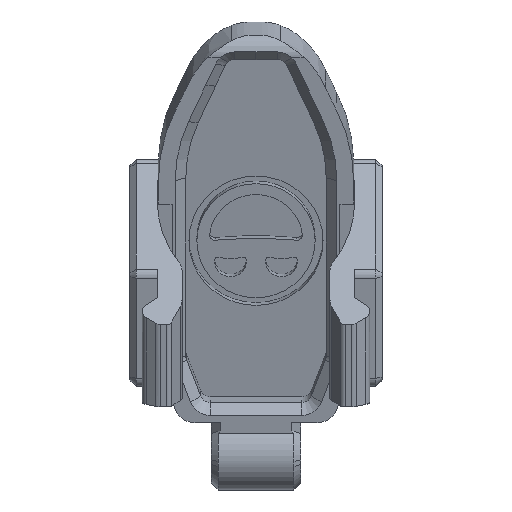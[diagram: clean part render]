
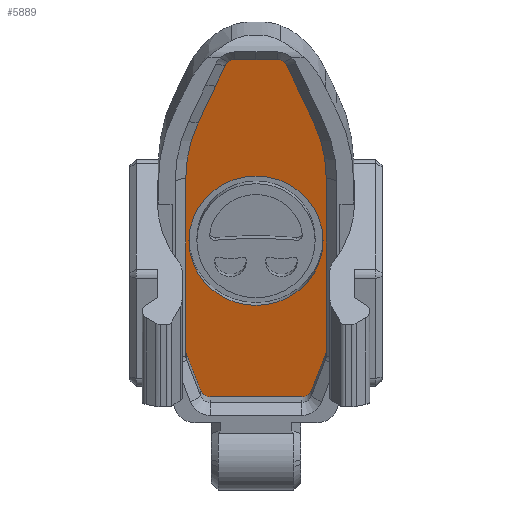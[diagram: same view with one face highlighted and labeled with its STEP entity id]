
A CAD part, top view. The second image highlights one B-rep face of the part: STEP entity #5889.
In plain terms, the highlighted planar face has unit normal (0, -0.266, 0.964).
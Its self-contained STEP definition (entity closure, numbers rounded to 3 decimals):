
#288=B_SPLINE_CURVE_WITH_KNOTS('',3,(#9458,#9459,#9460,#9461,#9462,#9463),
 .UNSPECIFIED.,.F.,.F.,(4,2,4),(0.,0.198,0.396),
 .UNSPECIFIED.);
#292=B_SPLINE_CURVE_WITH_KNOTS('',3,(#9488,#9489,#9490,#9491),
 .UNSPECIFIED.,.F.,.F.,(4,4),(-1.571,-1.141),
 .UNSPECIFIED.);
#359=B_SPLINE_CURVE_WITH_KNOTS('',3,(#11507,#11508,#11509,#11510,#11511,
#11512),.UNSPECIFIED.,.F.,.F.,(4,2,4),(0.,0.198,0.396),
 .UNSPECIFIED.);
#362=B_SPLINE_CURVE_WITH_KNOTS('',3,(#11533,#11534,#11535,#11536),
 .UNSPECIFIED.,.F.,.F.,(4,4),(-1.571,-1.141),
 .UNSPECIFIED.);
#551=LINE('',#9436,#1043);
#553=LINE('',#9494,#1045);
#557=LINE('',#9506,#1049);
#805=LINE('',#11489,#1297);
#809=LINE('',#11546,#1301);
#811=LINE('',#11555,#1303);
#818=LINE('',#11585,#1310);
#819=LINE('',#11607,#1311);
#1043=VECTOR('',#7022,10.);
#1045=VECTOR('',#7026,10.);
#1049=VECTOR('',#7038,10.);
#1297=VECTOR('',#7766,10.);
#1301=VECTOR('',#7772,10.);
#1303=VECTOR('',#7782,10.);
#1310=VECTOR('',#7817,10.);
#1311=VECTOR('',#7820,10.);
#1457=FACE_BOUND('',#2131,.T.);
#1763=FACE_OUTER_BOUND('',#2130,.T.);
#2130=EDGE_LOOP('',(#5178,#5179,#5180,#5181,#5182,#5183,#5184,#5185,#5186,
#5187,#5188,#5189,#5190,#5191,#5192,#5193,#5194,#5195));
#2131=EDGE_LOOP('',(#5196));
#2245=CIRCLE('',#6141,1.);
#2247=CIRCLE('',#6146,1.);
#2249=CIRCLE('',#6150,1.);
#2311=CIRCLE('',#6386,1.);
#2312=CIRCLE('',#6390,1.);
#2315=CIRCLE('',#6395,1.);
#2319=CIRCLE('',#6405,6.36);
#2528=VERTEX_POINT('',#9403);
#2529=VERTEX_POINT('',#9405);
#2533=VERTEX_POINT('',#9435);
#2534=VERTEX_POINT('',#9457);
#2537=VERTEX_POINT('',#9482);
#2538=VERTEX_POINT('',#9493);
#2541=VERTEX_POINT('',#9500);
#2542=VERTEX_POINT('',#9505);
#2545=VERTEX_POINT('',#9513);
#2804=VERTEX_POINT('',#11448);
#2805=VERTEX_POINT('',#11450);
#2809=VERTEX_POINT('',#11484);
#2810=VERTEX_POINT('',#11506);
#2813=VERTEX_POINT('',#11531);
#2815=VERTEX_POINT('',#11544);
#2817=VERTEX_POINT('',#11549);
#2818=VERTEX_POINT('',#11554);
#2821=VERTEX_POINT('',#11562);
#2823=VERTEX_POINT('',#11577);
#3162=EDGE_CURVE('',#2528,#2529,#2245,.T.);
#3168=EDGE_CURVE('',#2533,#2529,#551,.T.);
#3170=EDGE_CURVE('',#2534,#2533,#288,.F.);
#3175=EDGE_CURVE('',#2537,#2534,#292,.T.);
#3176=EDGE_CURVE('',#2538,#2537,#553,.T.);
#3181=EDGE_CURVE('',#2538,#2541,#2247,.T.);
#3182=EDGE_CURVE('',#2542,#2541,#557,.T.);
#3186=EDGE_CURVE('',#2542,#2545,#2249,.T.);
#3606=EDGE_CURVE('',#2805,#2804,#2311,.T.);
#3614=EDGE_CURVE('',#2809,#2804,#805,.T.);
#3615=EDGE_CURVE('',#2810,#2809,#359,.F.);
#3619=EDGE_CURVE('',#2813,#2810,#362,.T.);
#3623=EDGE_CURVE('',#2815,#2813,#809,.T.);
#3625=EDGE_CURVE('',#2815,#2817,#2312,.T.);
#3627=EDGE_CURVE('',#2818,#2817,#811,.T.);
#3632=EDGE_CURVE('',#2818,#2821,#2315,.T.);
#3638=EDGE_CURVE('',#2823,#2823,#2319,.T.);
#3641=EDGE_CURVE('',#2528,#2805,#818,.F.);
#3643=EDGE_CURVE('',#2545,#2821,#819,.T.);
#5178=ORIENTED_EDGE('',*,*,#3641,.T.);
#5179=ORIENTED_EDGE('',*,*,#3606,.T.);
#5180=ORIENTED_EDGE('',*,*,#3614,.F.);
#5181=ORIENTED_EDGE('',*,*,#3615,.F.);
#5182=ORIENTED_EDGE('',*,*,#3619,.F.);
#5183=ORIENTED_EDGE('',*,*,#3623,.F.);
#5184=ORIENTED_EDGE('',*,*,#3625,.T.);
#5185=ORIENTED_EDGE('',*,*,#3627,.F.);
#5186=ORIENTED_EDGE('',*,*,#3632,.T.);
#5187=ORIENTED_EDGE('',*,*,#3643,.F.);
#5188=ORIENTED_EDGE('',*,*,#3186,.F.);
#5189=ORIENTED_EDGE('',*,*,#3182,.T.);
#5190=ORIENTED_EDGE('',*,*,#3181,.F.);
#5191=ORIENTED_EDGE('',*,*,#3176,.T.);
#5192=ORIENTED_EDGE('',*,*,#3175,.T.);
#5193=ORIENTED_EDGE('',*,*,#3170,.T.);
#5194=ORIENTED_EDGE('',*,*,#3168,.T.);
#5195=ORIENTED_EDGE('',*,*,#3162,.F.);
#5196=ORIENTED_EDGE('',*,*,#3638,.T.);
#5560=PLANE('',#6408);
#5889=ADVANCED_FACE('',(#1763,#1457),#5560,.T.);
#6141=AXIS2_PLACEMENT_3D('',#9406,#7014,#7015);
#6146=AXIS2_PLACEMENT_3D('',#9503,#7034,#7035);
#6150=AXIS2_PLACEMENT_3D('',#9514,#7045,#7046);
#6386=AXIS2_PLACEMENT_3D('',#11451,#7758,#7759);
#6390=AXIS2_PLACEMENT_3D('',#11551,#7776,#7777);
#6395=AXIS2_PLACEMENT_3D('',#11564,#7790,#7791);
#6405=AXIS2_PLACEMENT_3D('',#11578,#7812,#7813);
#6408=AXIS2_PLACEMENT_3D('',#11609,#7822,#7823);
#7014=DIRECTION('center_axis',(0.,0.266,-0.964));
#7015=DIRECTION('ref_axis',(0.542,0.81,0.224));
#7022=DIRECTION('',(-0.412,0.878,0.243));
#7026=DIRECTION('',(0.,0.964,0.266));
#7034=DIRECTION('center_axis',(0.,0.266,-0.964));
#7035=DIRECTION('ref_axis',(0.984,-0.172,-0.048));
#7038=DIRECTION('',(0.352,0.902,0.249));
#7045=DIRECTION('center_axis',(0.,0.266,-0.964));
#7046=DIRECTION('ref_axis',(0.569,-0.793,-0.219));
#7758=DIRECTION('center_axis',(0.,-0.266,
0.964));
#7759=DIRECTION('ref_axis',(-0.542,0.81,0.224));
#7766=DIRECTION('',(0.412,0.878,0.243));
#7772=DIRECTION('',(0.,0.964,0.266));
#7776=DIRECTION('center_axis',(0.,-0.266,
0.964));
#7777=DIRECTION('ref_axis',(-0.984,-0.172,-0.048));
#7782=DIRECTION('',(-0.352,0.902,0.249));
#7790=DIRECTION('center_axis',(0.,-0.266,
0.964));
#7791=DIRECTION('ref_axis',(-0.569,-0.793,-0.219));
#7812=DIRECTION('center_axis',(0.,0.266,-0.964));
#7813=DIRECTION('ref_axis',(1.,0.,0.));
#7817=DIRECTION('',(1.,0.,0.));
#7820=DIRECTION('',(-1.,0.,0.));
#7822=DIRECTION('center_axis',(0.,-0.266,
0.964));
#7823=DIRECTION('ref_axis',(1.,0.,0.));
#9403=CARTESIAN_POINT('',(1.687,-87.656,-101.1));
#9405=CARTESIAN_POINT('',(2.598,-88.223,-101.256));
#9406=CARTESIAN_POINT('Origin',(1.687,-88.62,-101.366));
#9435=CARTESIAN_POINT('',(3.522,-90.194,-101.801));
#9436=CARTESIAN_POINT('',(7.188,-98.015,-103.96));
#9457=CARTESIAN_POINT('',(5.161,-93.672,-102.761));
#9458=CARTESIAN_POINT('Ctrl Pts',(3.522,-90.194,-101.801));
#9459=CARTESIAN_POINT('Ctrl Pts',(3.794,-90.774,-101.961));
#9460=CARTESIAN_POINT('Ctrl Pts',(4.066,-91.354,-102.121));
#9461=CARTESIAN_POINT('Ctrl Pts',(4.613,-92.513,-102.441));
#9462=CARTESIAN_POINT('Ctrl Pts',(4.886,-93.093,-102.601));
#9463=CARTESIAN_POINT('Ctrl Pts',(5.161,-93.672,-102.761));
#9482=CARTESIAN_POINT('',(6.337,-98.88,-104.198));
#9488=CARTESIAN_POINT('Ctrl Pts',(6.337,-98.88,-104.198));
#9489=CARTESIAN_POINT('Ctrl Pts',(6.337,-97.088,-103.704));
#9490=CARTESIAN_POINT('Ctrl Pts',(5.932,-95.3,-103.21));
#9491=CARTESIAN_POINT('Ctrl Pts',(5.161,-93.672,-102.761));
#9493=CARTESIAN_POINT('',(6.337,-115.792,-108.867));
#9494=CARTESIAN_POINT('',(6.337,-110.566,-107.425));
#9500=CARTESIAN_POINT('',(6.273,-116.131,-108.961));
#9503=CARTESIAN_POINT('Origin',(5.337,-115.792,-108.867));
#9505=CARTESIAN_POINT('',(4.934,-119.563,-109.908));
#9506=CARTESIAN_POINT('',(7.25,-113.626,-108.269));
#9513=CARTESIAN_POINT('',(3.998,-120.188,-110.081));
#9514=CARTESIAN_POINT('Origin',(3.998,-119.224,-109.815));
#11448=CARTESIAN_POINT('',(-3.251,-88.223,-101.256));
#11450=CARTESIAN_POINT('',(-2.34,-87.656,-101.1));
#11451=CARTESIAN_POINT('Origin',(-2.34,-88.62,-101.366));
#11484=CARTESIAN_POINT('',(-4.175,-90.194,-101.801));
#11489=CARTESIAN_POINT('',(-7.841,-98.015,-103.96));
#11506=CARTESIAN_POINT('',(-5.814,-93.672,-102.761));
#11507=CARTESIAN_POINT('Ctrl Pts',(-4.175,-90.194,
-101.801));
#11508=CARTESIAN_POINT('Ctrl Pts',(-4.447,-90.774,
-101.961));
#11509=CARTESIAN_POINT('Ctrl Pts',(-4.719,-91.354,
-102.121));
#11510=CARTESIAN_POINT('Ctrl Pts',(-5.266,-92.513,-102.441));
#11511=CARTESIAN_POINT('Ctrl Pts',(-5.539,-93.093,
-102.601));
#11512=CARTESIAN_POINT('Ctrl Pts',(-5.814,-93.672,
-102.761));
#11531=CARTESIAN_POINT('',(-6.99,-98.88,-104.198));
#11533=CARTESIAN_POINT('Ctrl Pts',(-6.99,-98.88,
-104.198));
#11534=CARTESIAN_POINT('Ctrl Pts',(-6.99,-97.088,
-103.704));
#11535=CARTESIAN_POINT('Ctrl Pts',(-6.585,-95.3,-103.21));
#11536=CARTESIAN_POINT('Ctrl Pts',(-5.814,-93.672,-102.761));
#11544=CARTESIAN_POINT('',(-6.99,-115.792,-108.867));
#11546=CARTESIAN_POINT('',(-6.99,-110.566,-107.425));
#11549=CARTESIAN_POINT('',(-6.926,-116.131,-108.961));
#11551=CARTESIAN_POINT('Origin',(-5.99,-115.792,-108.867));
#11554=CARTESIAN_POINT('',(-5.587,-119.563,-109.908));
#11555=CARTESIAN_POINT('',(-7.903,-113.626,-108.269));
#11562=CARTESIAN_POINT('',(-4.651,-120.188,-110.081));
#11564=CARTESIAN_POINT('Origin',(-4.651,-119.224,-109.815));
#11577=CARTESIAN_POINT('',(-6.687,-105.368,-105.99));
#11578=CARTESIAN_POINT('Origin',(-0.327,-105.368,-105.99));
#11585=CARTESIAN_POINT('',(3.269,-87.656,-101.1));
#11607=CARTESIAN_POINT('',(-2.642,-120.188,-110.081));
#11609=CARTESIAN_POINT('Origin',(-4.958,-104.912,-105.864));
